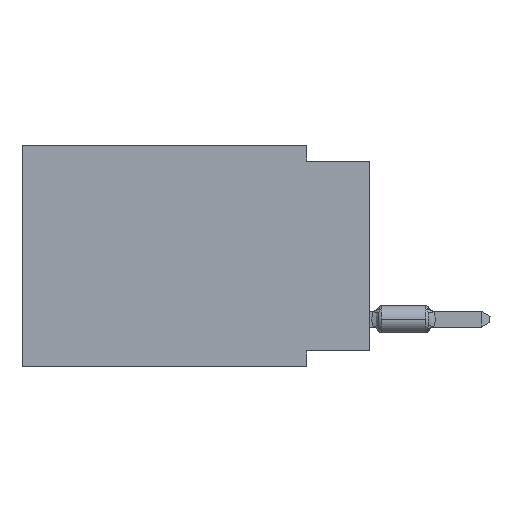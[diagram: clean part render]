
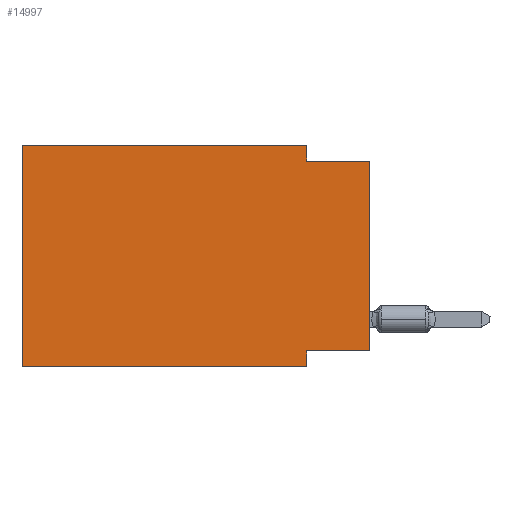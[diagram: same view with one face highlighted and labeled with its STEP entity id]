
A CAD part, left-side view. The second image highlights one B-rep face of the part: STEP entity #14997.
In plain terms, the highlighted planar face has unit normal (-1, 0, 0).
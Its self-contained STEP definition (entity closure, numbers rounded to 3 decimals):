
#255 = EDGE_CURVE ( 'NONE', #23369, #5222, #34835, .T. ) ;
#908 = CARTESIAN_POINT ( 'NONE',  ( 0., 13.97, 0. ) ) ;
#1109 = VECTOR ( 'NONE', #7928, 1000. ) ;
#1471 = VERTEX_POINT ( 'NONE', #13770 ) ;
#2048 = LINE ( 'NONE', #51296, #43316 ) ;
#3375 = LINE ( 'NONE', #42750, #14453 ) ;
#3453 = DIRECTION ( 'NONE',  ( 0., 1., 0. ) ) ;
#3778 = CARTESIAN_POINT ( 'NONE',  ( 0., 0., -8.255 ) ) ;
#5222 = VERTEX_POINT ( 'NONE', #27843 ) ;
#7928 = DIRECTION ( 'NONE',  ( 0., 0., 1. ) ) ;
#8168 = DIRECTION ( 'NONE',  ( 0., 0., 1. ) ) ;
#8232 = LINE ( 'NONE', #22338, #1109 ) ;
#9232 = DIRECTION ( 'NONE',  ( 0., 0., -1. ) ) ;
#9761 = DIRECTION ( 'NONE',  ( 0., 0., -1. ) ) ;
#10238 = EDGE_CURVE ( 'NONE', #44096, #12953, #54325, .T. ) ;
#10702 = VECTOR ( 'NONE', #45816, 1000. ) ;
#11413 = FACE_OUTER_BOUND ( 'NONE', #58507, .T. ) ;
#11471 = EDGE_CURVE ( 'NONE', #36208, #23369, #37394, .T. ) ;
#12953 = VERTEX_POINT ( 'NONE', #53049 ) ;
#13015 = VERTEX_POINT ( 'NONE', #24564 ) ;
#13535 = EDGE_CURVE ( 'NONE', #12953, #13015, #53591, .T. ) ;
#13770 = CARTESIAN_POINT ( 'NONE',  ( 0., 0., -0.635 ) ) ;
#14453 = VECTOR ( 'NONE', #8168, 1000. ) ;
#14478 = ORIENTED_EDGE ( 'NONE', *, *, #38121, .F. ) ;
#14997 = ADVANCED_FACE ( 'NONE', ( #11413 ), #36049, .F. ) ;
#15747 = CARTESIAN_POINT ( 'NONE',  ( 0., 13.97, -8.89 ) ) ;
#16397 = CARTESIAN_POINT ( 'NONE',  ( 0., 13.97, 0. ) ) ;
#17690 = EDGE_CURVE ( 'NONE', #54451, #5222, #55713, .T. ) ;
#19248 = ORIENTED_EDGE ( 'NONE', *, *, #255, .F. ) ;
#20415 = DIRECTION ( 'NONE',  ( 0., -1., 0. ) ) ;
#21079 = ORIENTED_EDGE ( 'NONE', *, *, #13535, .F. ) ;
#22338 = CARTESIAN_POINT ( 'NONE',  ( 0., 0., 0. ) ) ;
#23369 = VERTEX_POINT ( 'NONE', #26491 ) ;
#24483 = ORIENTED_EDGE ( 'NONE', *, *, #35454, .F. ) ;
#24564 = CARTESIAN_POINT ( 'NONE',  ( 0., 2.54, -0.635 ) ) ;
#26491 = CARTESIAN_POINT ( 'NONE',  ( 0., 2.54, -8.255 ) ) ;
#27843 = CARTESIAN_POINT ( 'NONE',  ( 0., 2.54, -8.89 ) ) ;
#33462 = CARTESIAN_POINT ( 'NONE',  ( 0., 2.54, 0. ) ) ;
#34835 = LINE ( 'NONE', #58814, #50316 ) ;
#35454 = EDGE_CURVE ( 'NONE', #54451, #44096, #3375, .T. ) ;
#36049 = PLANE ( 'NONE',  #49936 ) ;
#36208 = VERTEX_POINT ( 'NONE', #41259 ) ;
#37394 = LINE ( 'NONE', #3778, #44171 ) ;
#38121 = EDGE_CURVE ( 'NONE', #13015, #1471, #2048, .T. ) ;
#38154 = ORIENTED_EDGE ( 'NONE', *, *, #48596, .T. ) ;
#38380 = ORIENTED_EDGE ( 'NONE', *, *, #10238, .F. ) ;
#41259 = CARTESIAN_POINT ( 'NONE',  ( 0., 0., -8.255 ) ) ;
#42750 = CARTESIAN_POINT ( 'NONE',  ( 0., 13.97, 0. ) ) ;
#43316 = VECTOR ( 'NONE', #55789, 1000. ) ;
#44080 = VECTOR ( 'NONE', #20415, 1000. ) ;
#44096 = VERTEX_POINT ( 'NONE', #16397 ) ;
#44171 = VECTOR ( 'NONE', #3453, 1000. ) ;
#45816 = DIRECTION ( 'NONE',  ( 0., -1., 0. ) ) ;
#48596 = EDGE_CURVE ( 'NONE', #36208, #1471, #8232, .T. ) ;
#49936 = AXIS2_PLACEMENT_3D ( 'NONE', #50760, #56164, #50129 ) ;
#50129 = DIRECTION ( 'NONE',  ( 0., 0., -1. ) ) ;
#50316 = VECTOR ( 'NONE', #9232, 1000. ) ;
#50760 = CARTESIAN_POINT ( 'NONE',  ( 0., 13.97, 0. ) ) ;
#51296 = CARTESIAN_POINT ( 'NONE',  ( 0., 0., -0.635 ) ) ;
#51484 = ORIENTED_EDGE ( 'NONE', *, *, #11471, .F. ) ;
#53049 = CARTESIAN_POINT ( 'NONE',  ( 0., 2.54, 0. ) ) ;
#53591 = LINE ( 'NONE', #33462, #56893 ) ;
#54325 = LINE ( 'NONE', #908, #44080 ) ;
#54451 = VERTEX_POINT ( 'NONE', #60265 ) ;
#55713 = LINE ( 'NONE', #15747, #10702 ) ;
#55789 = DIRECTION ( 'NONE',  ( 0., -1., 0. ) ) ;
#56164 = DIRECTION ( 'NONE',  ( 1., 0., 0. ) ) ;
#56893 = VECTOR ( 'NONE', #9761, 1000. ) ;
#58507 = EDGE_LOOP ( 'NONE', ( #38154, #14478, #21079, #38380, #24483, #61874, #19248, #51484 ) ) ;
#58814 = CARTESIAN_POINT ( 'NONE',  ( 0., 2.54, -8.89 ) ) ;
#60265 = CARTESIAN_POINT ( 'NONE',  ( 0., 13.97, -8.89 ) ) ;
#61874 = ORIENTED_EDGE ( 'NONE', *, *, #17690, .T. ) ;
